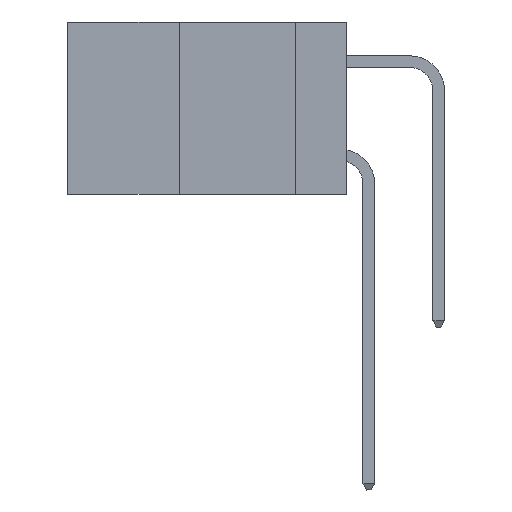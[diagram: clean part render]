
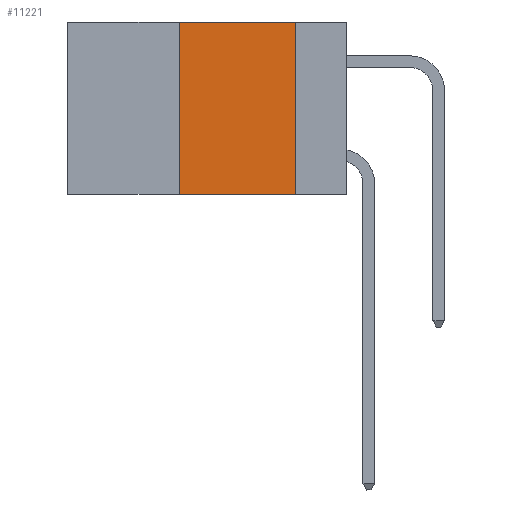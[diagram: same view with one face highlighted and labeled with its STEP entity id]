
A CAD part, left-side view. The second image highlights one B-rep face of the part: STEP entity #11221.
In plain terms, the highlighted planar face has unit normal (-1, 0, 0).
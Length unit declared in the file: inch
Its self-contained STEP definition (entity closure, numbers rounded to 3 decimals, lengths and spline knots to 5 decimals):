
#21 = CARTESIAN_POINT ( 'NONE',  ( 0., 0.36, 0. ) ) ;
#235 = EDGE_CURVE ( 'NONE', #4750, #9781, #12186, .T. ) ;
#929 = VERTEX_POINT ( 'NONE', #21 ) ;
#1295 = CARTESIAN_POINT ( 'NONE',  ( 0., 0.36, 0. ) ) ;
#1345 = DIRECTION ( 'NONE',  ( 0., 0., -1. ) ) ;
#1450 = CARTESIAN_POINT ( 'NONE',  ( 0., 0.6, 0. ) ) ;
#1821 = EDGE_CURVE ( 'NONE', #929, #4273, #2870, .T. ) ;
#2870 = LINE ( 'NONE', #1450, #7733 ) ;
#3160 = DIRECTION ( 'NONE',  ( 0., 0., -1. ) ) ;
#3194 = CARTESIAN_POINT ( 'NONE',  ( 0., 0.6, 0. ) ) ;
#3313 = PLANE ( 'NONE',  #5155 ) ;
#3363 = DIRECTION ( 'NONE',  ( 0., -1., 0. ) ) ;
#3982 = FACE_OUTER_BOUND ( 'NONE', #9482, .T. ) ;
#4033 = ORIENTED_EDGE ( 'NONE', *, *, #8487, .F. ) ;
#4273 = VERTEX_POINT ( 'NONE', #10649 ) ;
#4328 = VECTOR ( 'NONE', #1345, 39.37008 ) ;
#4408 = CARTESIAN_POINT ( 'NONE',  ( 0., 0.11, -0.37 ) ) ;
#4609 = ORIENTED_EDGE ( 'NONE', *, *, #1821, .F. ) ;
#4750 = VERTEX_POINT ( 'NONE', #10493 ) ;
#5155 = AXIS2_PLACEMENT_3D ( 'NONE', #3194, #10112, #3160 ) ;
#5185 = VECTOR ( 'NONE', #3363, 39.37008 ) ;
#5738 = DIRECTION ( 'NONE',  ( 0., -1., 0. ) ) ;
#5839 = ORIENTED_EDGE ( 'NONE', *, *, #235, .T. ) ;
#5885 = LINE ( 'NONE', #1295, #9987 ) ;
#6217 = CARTESIAN_POINT ( 'NONE',  ( 0., 0.11, 0. ) ) ;
#7235 = EDGE_CURVE ( 'NONE', #4750, #929, #5885, .T. ) ;
#7691 = ORIENTED_EDGE ( 'NONE', *, *, #7235, .F. ) ;
#7733 = VECTOR ( 'NONE', #5738, 39.37008 ) ;
#8138 = DIRECTION ( 'NONE',  ( 0., 0., 1. ) ) ;
#8487 = EDGE_CURVE ( 'NONE', #4273, #9781, #9015, .T. ) ;
#9015 = LINE ( 'NONE', #6217, #4328 ) ;
#9482 = EDGE_LOOP ( 'NONE', ( #4033, #4609, #7691, #5839 ) ) ;
#9781 = VERTEX_POINT ( 'NONE', #4408 ) ;
#9987 = VECTOR ( 'NONE', #8138, 39.37008 ) ;
#10039 = CARTESIAN_POINT ( 'NONE',  ( 0., 0.6, -0.37 ) ) ;
#10112 = DIRECTION ( 'NONE',  ( 1., 0., 0. ) ) ;
#10493 = CARTESIAN_POINT ( 'NONE',  ( 0., 0.36, -0.37 ) ) ;
#10649 = CARTESIAN_POINT ( 'NONE',  ( 0., 0.11, 0. ) ) ;
#11221 = ADVANCED_FACE ( 'NONE', ( #3982 ), #3313, .F. ) ;
#12186 = LINE ( 'NONE', #10039, #5185 ) ;
